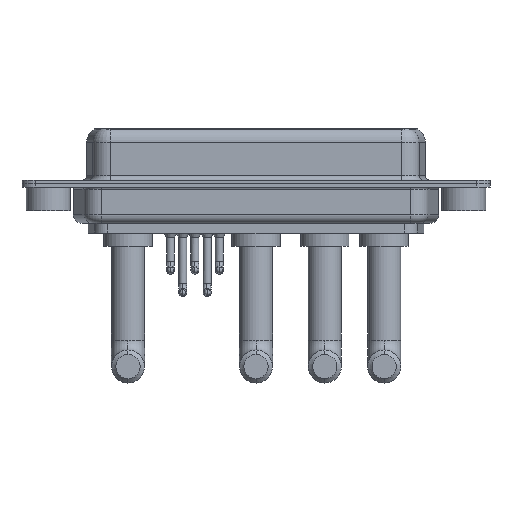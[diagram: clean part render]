
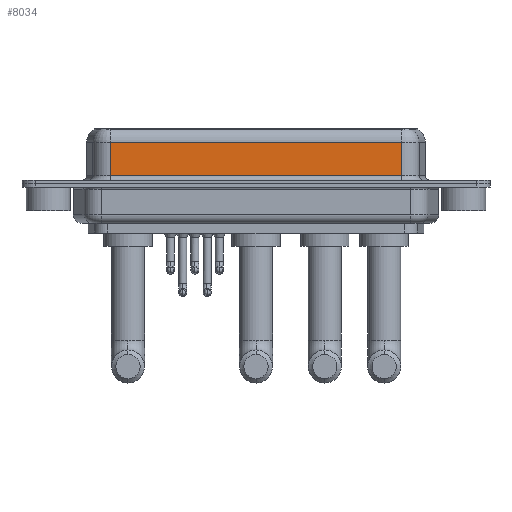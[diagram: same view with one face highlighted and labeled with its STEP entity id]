
A CAD part, front view. The second image highlights one B-rep face of the part: STEP entity #8034.
In plain terms, the highlighted planar face has unit normal (0, -1, 0).
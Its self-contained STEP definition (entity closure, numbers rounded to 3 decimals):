
#234 = EDGE_LOOP ( 'NONE', ( #16198, #5965, #6325, #17219 ) ) ;
#576 = EDGE_CURVE ( 'NONE', #16444, #9004, #6626, .T. ) ;
#820 = LINE ( 'NONE', #9836, #3258 ) ;
#1016 = EDGE_CURVE ( 'NONE', #15676, #16265, #15086, .T. ) ;
#1653 = LINE ( 'NONE', #1834, #4527 ) ;
#1834 = CARTESIAN_POINT ( 'NONE',  ( 40.037, -3.95, 0.9 ) ) ;
#2047 = DIRECTION ( 'NONE',  ( -1., 0., 0. ) ) ;
#3258 = VECTOR ( 'NONE', #2047, 1000. ) ;
#3307 = CARTESIAN_POINT ( 'NONE',  ( 7.013, -3.95, 4.65 ) ) ;
#4384 = CARTESIAN_POINT ( 'NONE',  ( 7.013, -3.95, 0.9 ) ) ;
#4527 = VECTOR ( 'NONE', #11176, 1000. ) ;
#5388 = AXIS2_PLACEMENT_3D ( 'NONE', #9426, #8285, #13603 ) ;
#5965 = ORIENTED_EDGE ( 'NONE', *, *, #12694, .T. ) ;
#5979 = VECTOR ( 'NONE', #12099, 1000. ) ;
#6321 = EDGE_CURVE ( 'NONE', #16265, #9004, #1653, .T. ) ;
#6325 = ORIENTED_EDGE ( 'NONE', *, *, #1016, .T. ) ;
#6540 = CARTESIAN_POINT ( 'NONE',  ( 40.037, -3.95, 6.4 ) ) ;
#6626 = LINE ( 'NONE', #6540, #16041 ) ;
#8034 = ADVANCED_FACE ( 'NONE', ( #9255 ), #13243, .F. ) ;
#8285 = DIRECTION ( 'NONE',  ( 0., 1., 0. ) ) ;
#9004 = VERTEX_POINT ( 'NONE', #9013 ) ;
#9013 = CARTESIAN_POINT ( 'NONE',  ( 40.037, -3.95, 0.9 ) ) ;
#9242 = DIRECTION ( 'NONE',  ( 0., 0., -1. ) ) ;
#9255 = FACE_OUTER_BOUND ( 'NONE', #234, .T. ) ;
#9426 = CARTESIAN_POINT ( 'NONE',  ( 40.037, -3.95, 6.4 ) ) ;
#9836 = CARTESIAN_POINT ( 'NONE',  ( 40.037, -3.95, 4.65 ) ) ;
#11176 = DIRECTION ( 'NONE',  ( 1., 0., 0. ) ) ;
#12099 = DIRECTION ( 'NONE',  ( 0., 0., -1. ) ) ;
#12694 = EDGE_CURVE ( 'NONE', #16444, #15676, #820, .T. ) ;
#13243 = PLANE ( 'NONE',  #5388 ) ;
#13603 = DIRECTION ( 'NONE',  ( 0., 0., 1. ) ) ;
#14823 = CARTESIAN_POINT ( 'NONE',  ( 7.013, -3.95, 6.4 ) ) ;
#15086 = LINE ( 'NONE', #14823, #5979 ) ;
#15566 = CARTESIAN_POINT ( 'NONE',  ( 40.037, -3.95, 4.65 ) ) ;
#15676 = VERTEX_POINT ( 'NONE', #3307 ) ;
#16041 = VECTOR ( 'NONE', #9242, 1000. ) ;
#16198 = ORIENTED_EDGE ( 'NONE', *, *, #576, .F. ) ;
#16265 = VERTEX_POINT ( 'NONE', #4384 ) ;
#16444 = VERTEX_POINT ( 'NONE', #15566 ) ;
#17219 = ORIENTED_EDGE ( 'NONE', *, *, #6321, .T. ) ;
